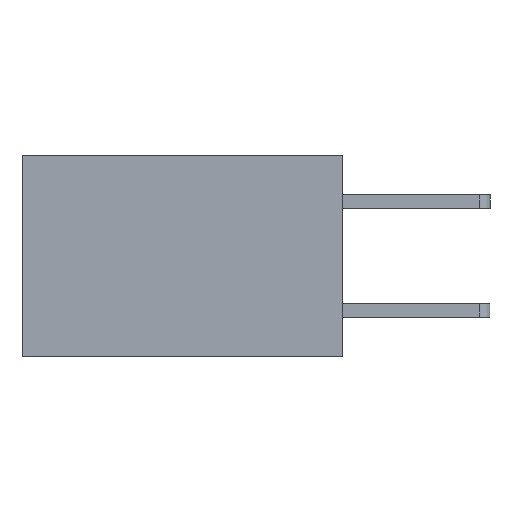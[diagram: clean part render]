
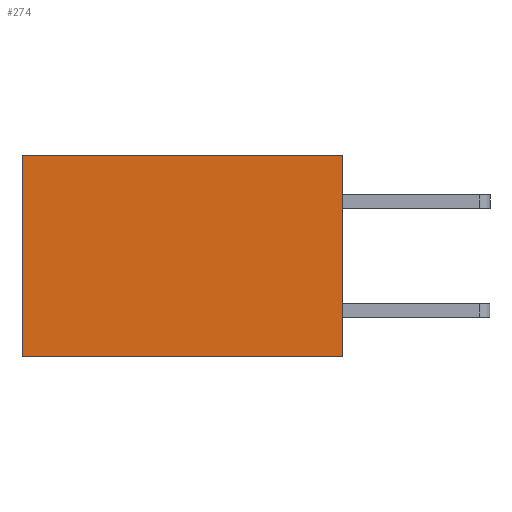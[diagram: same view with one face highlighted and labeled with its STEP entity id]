
A CAD part, left-side view. The second image highlights one B-rep face of the part: STEP entity #274.
In plain terms, the highlighted planar face has unit normal (-1, 0, 0).
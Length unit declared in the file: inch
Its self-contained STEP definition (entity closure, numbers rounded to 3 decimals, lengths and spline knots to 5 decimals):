
#160 = LINE ( 'NONE', #3383, #1940 ) ;
#274 = ADVANCED_FACE ( 'NONE', ( #850 ), #3760, .F. ) ;
#603 = VERTEX_POINT ( 'NONE', #7021 ) ;
#850 = FACE_OUTER_BOUND ( 'NONE', #2459, .T. ) ;
#1250 = VERTEX_POINT ( 'NONE', #7901 ) ;
#1940 = VECTOR ( 'NONE', #3483, 39.37008 ) ;
#2092 = ORIENTED_EDGE ( 'NONE', *, *, #5913, .T. ) ;
#2100 = ORIENTED_EDGE ( 'NONE', *, *, #6203, .F. ) ;
#2112 = ORIENTED_EDGE ( 'NONE', *, *, #4508, .F. ) ;
#2120 = ORIENTED_EDGE ( 'NONE', *, *, #2999, .T. ) ;
#2459 = EDGE_LOOP ( 'NONE', ( #2092, #2100, #2112, #2120 ) ) ;
#2512 = VECTOR ( 'NONE', #7828, 39.37008 ) ;
#2999 = EDGE_CURVE ( 'NONE', #4318, #603, #6816, .T. ) ;
#3284 = VECTOR ( 'NONE', #4215, 39.37008 ) ;
#3289 = VERTEX_POINT ( 'NONE', #7780 ) ;
#3383 = CARTESIAN_POINT ( 'NONE',  ( 0.277, 0.59, -0.37 ) ) ;
#3483 = DIRECTION ( 'NONE',  ( 0., 0., -1. ) ) ;
#3659 = DIRECTION ( 'NONE',  ( 0., 0., -1. ) ) ;
#3760 = PLANE ( 'NONE',  #7660 ) ;
#3770 = DIRECTION ( 'NONE',  ( 1., 0., 0. ) ) ;
#4098 = LINE ( 'NONE', #7831, #2512 ) ;
#4215 = DIRECTION ( 'NONE',  ( 0., 0., -1. ) ) ;
#4318 = VERTEX_POINT ( 'NONE', #5898 ) ;
#4508 = EDGE_CURVE ( 'NONE', #4318, #1250, #4872, .T. ) ;
#4695 = CARTESIAN_POINT ( 'NONE',  ( 0.277, 0., -0.37 ) ) ;
#4872 = LINE ( 'NONE', #4695, #3284 ) ;
#5364 = VECTOR ( 'NONE', #6179, 39.37008 ) ;
#5898 = CARTESIAN_POINT ( 'NONE',  ( 0.277, 0., 0. ) ) ;
#5913 = EDGE_CURVE ( 'NONE', #603, #3289, #160, .T. ) ;
#6179 = DIRECTION ( 'NONE',  ( 0., 1., 0. ) ) ;
#6203 = EDGE_CURVE ( 'NONE', #1250, #3289, #4098, .T. ) ;
#6732 = CARTESIAN_POINT ( 'NONE',  ( 0.277, 0., -0.37 ) ) ;
#6816 = LINE ( 'NONE', #7833, #5364 ) ;
#7021 = CARTESIAN_POINT ( 'NONE',  ( 0.277, 0.59, 0. ) ) ;
#7660 = AXIS2_PLACEMENT_3D ( 'NONE', #6732, #3770, #3659 ) ;
#7780 = CARTESIAN_POINT ( 'NONE',  ( 0.277, 0.59, -0.37 ) ) ;
#7828 = DIRECTION ( 'NONE',  ( 0., 1., 0. ) ) ;
#7831 = CARTESIAN_POINT ( 'NONE',  ( 0.277, 0., -0.37 ) ) ;
#7833 = CARTESIAN_POINT ( 'NONE',  ( 0.277, 0., 0. ) ) ;
#7901 = CARTESIAN_POINT ( 'NONE',  ( 0.277, 0., -0.37 ) ) ;
